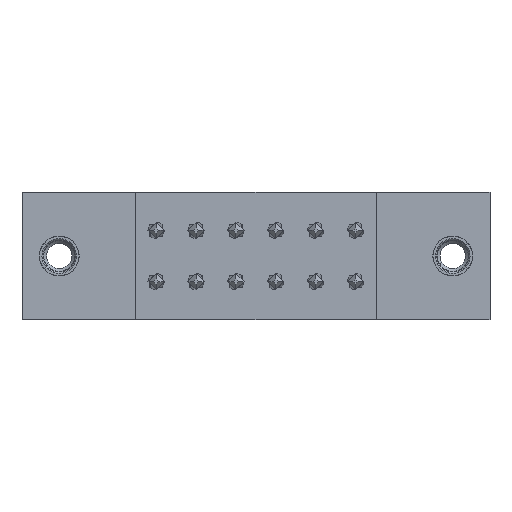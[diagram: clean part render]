
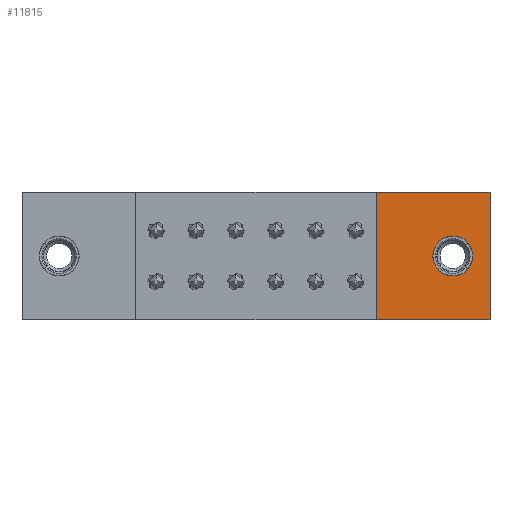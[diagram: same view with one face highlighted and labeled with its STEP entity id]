
A CAD part, front view. The second image highlights one B-rep face of the part: STEP entity #11815.
In plain terms, the highlighted planar face has unit normal (0, -1, 0).
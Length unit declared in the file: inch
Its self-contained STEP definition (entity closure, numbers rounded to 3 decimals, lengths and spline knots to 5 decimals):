
#69 = DIRECTION ( 'NONE',  ( 0., 0., -1. ) ) ;
#423 = EDGE_CURVE ( 'NONE', #14190, #8328, #13348, .T. ) ;
#580 = LINE ( 'NONE', #7855, #14072 ) ;
#644 = PLANE ( 'NONE',  #4368 ) ;
#1070 = CARTESIAN_POINT ( 'NONE',  ( 1.83, 0.163, 0. ) ) ;
#1448 = ORIENTED_EDGE ( 'NONE', *, *, #13755, .T. ) ;
#1721 = LINE ( 'NONE', #1070, #13224 ) ;
#2218 = ORIENTED_EDGE ( 'NONE', *, *, #423, .T. ) ;
#2437 = ORIENTED_EDGE ( 'NONE', *, *, #2445, .T. ) ;
#2445 = EDGE_CURVE ( 'NONE', #2871, #11142, #580, .T. ) ;
#2871 = VERTEX_POINT ( 'NONE', #3167 ) ;
#2961 = CARTESIAN_POINT ( 'NONE',  ( 1.83, 0.163, -0.5 ) ) ;
#3167 = CARTESIAN_POINT ( 'NONE',  ( 1.385, 0.163, 0. ) ) ;
#3537 = DIRECTION ( 'NONE',  ( -1., 0., 0. ) ) ;
#3577 = FACE_OUTER_BOUND ( 'NONE', #12825, .T. ) ;
#4085 = EDGE_CURVE ( 'NONE', #9866, #12345, #11334, .T. ) ;
#4368 = AXIS2_PLACEMENT_3D ( 'NONE', #8608, #11073, #6392 ) ;
#4467 = LINE ( 'NONE', #9676, #7157 ) ;
#4633 = DIRECTION ( 'NONE',  ( 0., 1., 0. ) ) ;
#5062 = CARTESIAN_POINT ( 'NONE',  ( 1.385, 0.163, -0.5 ) ) ;
#5078 = EDGE_CURVE ( 'NONE', #11142, #9866, #4467, .T. ) ;
#5129 = CARTESIAN_POINT ( 'NONE',  ( 1.83, 0.163, 0. ) ) ;
#5177 = ORIENTED_EDGE ( 'NONE', *, *, #10255, .T. ) ;
#6392 = DIRECTION ( 'NONE',  ( 0., 0., -1. ) ) ;
#6601 = CARTESIAN_POINT ( 'NONE',  ( 1.6845, 0.163, -0.25 ) ) ;
#6709 = DIRECTION ( 'NONE',  ( 0., 0., 1. ) ) ;
#7157 = VECTOR ( 'NONE', #10737, 39.37008 ) ;
#7280 = CARTESIAN_POINT ( 'NONE',  ( 1.6845, 0.163, -0.172 ) ) ;
#7655 = DIRECTION ( 'NONE',  ( 0., 1., 0. ) ) ;
#7855 = CARTESIAN_POINT ( 'NONE',  ( 1.385, 0.163, -0.5 ) ) ;
#8328 = VERTEX_POINT ( 'NONE', #7280 ) ;
#8463 = VECTOR ( 'NONE', #6709, 39.37008 ) ;
#8608 = CARTESIAN_POINT ( 'NONE',  ( 1.83, 0.163, 0. ) ) ;
#8781 = CARTESIAN_POINT ( 'NONE',  ( 1.6845, 0.163, -0.328 ) ) ;
#9365 = EDGE_LOOP ( 'NONE', ( #5177, #2218 ) ) ;
#9676 = CARTESIAN_POINT ( 'NONE',  ( 1.83, 0.163, -0.5 ) ) ;
#9866 = VERTEX_POINT ( 'NONE', #2961 ) ;
#10255 = EDGE_CURVE ( 'NONE', #8328, #14190, #13296, .T. ) ;
#10737 = DIRECTION ( 'NONE',  ( 1., 0., 0. ) ) ;
#10941 = FACE_BOUND ( 'NONE', #9365, .T. ) ;
#10972 = AXIS2_PLACEMENT_3D ( 'NONE', #6601, #7655, #12233 ) ;
#11073 = DIRECTION ( 'NONE',  ( 0., -1., 0. ) ) ;
#11142 = VERTEX_POINT ( 'NONE', #5062 ) ;
#11334 = LINE ( 'NONE', #13553, #8463 ) ;
#11395 = DIRECTION ( 'NONE',  ( 0., 0., -1. ) ) ;
#11610 = ORIENTED_EDGE ( 'NONE', *, *, #4085, .T. ) ;
#11815 = ADVANCED_FACE ( 'NONE', ( #3577, #10941 ), #644, .T. ) ;
#12233 = DIRECTION ( 'NONE',  ( 0., 0., -1. ) ) ;
#12345 = VERTEX_POINT ( 'NONE', #5129 ) ;
#12731 = CARTESIAN_POINT ( 'NONE',  ( 1.6845, 0.163, -0.25 ) ) ;
#12825 = EDGE_LOOP ( 'NONE', ( #11610, #1448, #2437, #13114 ) ) ;
#13114 = ORIENTED_EDGE ( 'NONE', *, *, #5078, .T. ) ;
#13224 = VECTOR ( 'NONE', #3537, 39.37008 ) ;
#13296 = CIRCLE ( 'NONE', #13508, 0.078 ) ;
#13348 = CIRCLE ( 'NONE', #10972, 0.078 ) ;
#13508 = AXIS2_PLACEMENT_3D ( 'NONE', #12731, #4633, #69 ) ;
#13553 = CARTESIAN_POINT ( 'NONE',  ( 1.83, 0.163, -0.5 ) ) ;
#13755 = EDGE_CURVE ( 'NONE', #12345, #2871, #1721, .T. ) ;
#14072 = VECTOR ( 'NONE', #11395, 39.37008 ) ;
#14190 = VERTEX_POINT ( 'NONE', #8781 ) ;
